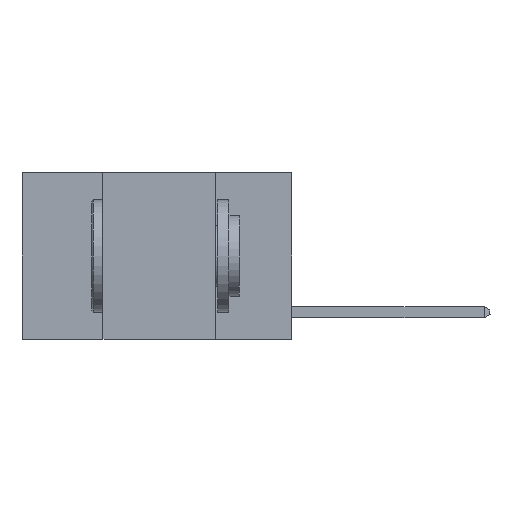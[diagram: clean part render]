
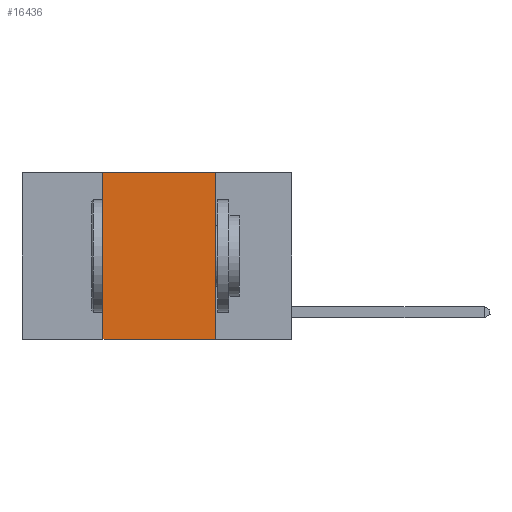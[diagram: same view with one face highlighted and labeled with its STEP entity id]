
A CAD part, left-side view. The second image highlights one B-rep face of the part: STEP entity #16436.
In plain terms, the highlighted planar face has unit normal (-1, 0, 0).
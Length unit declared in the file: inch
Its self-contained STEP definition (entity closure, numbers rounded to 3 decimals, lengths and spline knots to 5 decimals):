
#445 = VECTOR ( 'NONE', #25201, 39.37008 ) ;
#454 = ORIENTED_EDGE ( 'NONE', *, *, #23376, .F. ) ;
#1463 = PLANE ( 'NONE',  #14827 ) ;
#1881 = EDGE_CURVE ( 'NONE', #23136, #19070, #21508, .T. ) ;
#3064 = VERTEX_POINT ( 'NONE', #17737 ) ;
#4097 = LINE ( 'NONE', #4528, #22938 ) ;
#4528 = CARTESIAN_POINT ( 'NONE',  ( 0., 0.6, -0.37 ) ) ;
#6183 = VECTOR ( 'NONE', #24959, 39.37008 ) ;
#6188 = CARTESIAN_POINT ( 'NONE',  ( 0., 0.6, 0. ) ) ;
#7070 = ORIENTED_EDGE ( 'NONE', *, *, #15019, .T. ) ;
#8192 = CARTESIAN_POINT ( 'NONE',  ( 0., 0.17, -0.37 ) ) ;
#10512 = EDGE_CURVE ( 'NONE', #3064, #15084, #11759, .T. ) ;
#10969 = ORIENTED_EDGE ( 'NONE', *, *, #10512, .F. ) ;
#11759 = LINE ( 'NONE', #22546, #445 ) ;
#12192 = CARTESIAN_POINT ( 'NONE',  ( 0., 0.42, 0. ) ) ;
#13046 = DIRECTION ( 'NONE',  ( 1., 0., 0. ) ) ;
#14827 = AXIS2_PLACEMENT_3D ( 'NONE', #6188, #13046, #22053 ) ;
#15019 = EDGE_CURVE ( 'NONE', #3064, #19070, #4097, .T. ) ;
#15084 = VERTEX_POINT ( 'NONE', #12192 ) ;
#15989 = DIRECTION ( 'NONE',  ( 0., -1., 0. ) ) ;
#16436 = ADVANCED_FACE ( 'NONE', ( #26482 ), #1463, .F. ) ;
#17418 = ORIENTED_EDGE ( 'NONE', *, *, #1881, .F. ) ;
#17737 = CARTESIAN_POINT ( 'NONE',  ( 0., 0.42, -0.37 ) ) ;
#18184 = CARTESIAN_POINT ( 'NONE',  ( 0., 0.6, 0. ) ) ;
#19070 = VERTEX_POINT ( 'NONE', #8192 ) ;
#19665 = CARTESIAN_POINT ( 'NONE',  ( 0., 0.17, 0. ) ) ;
#20391 = LINE ( 'NONE', #18184, #6183 ) ;
#21508 = LINE ( 'NONE', #25485, #25277 ) ;
#22053 = DIRECTION ( 'NONE',  ( 0., 0., -1. ) ) ;
#22546 = CARTESIAN_POINT ( 'NONE',  ( 0., 0.42, 0. ) ) ;
#22894 = EDGE_LOOP ( 'NONE', ( #17418, #454, #10969, #7070 ) ) ;
#22938 = VECTOR ( 'NONE', #15989, 39.37008 ) ;
#23136 = VERTEX_POINT ( 'NONE', #19665 ) ;
#23376 = EDGE_CURVE ( 'NONE', #15084, #23136, #20391, .T. ) ;
#24959 = DIRECTION ( 'NONE',  ( 0., -1., 0. ) ) ;
#25201 = DIRECTION ( 'NONE',  ( 0., 0., 1. ) ) ;
#25277 = VECTOR ( 'NONE', #27839, 39.37008 ) ;
#25485 = CARTESIAN_POINT ( 'NONE',  ( 0., 0.17, 0. ) ) ;
#26482 = FACE_OUTER_BOUND ( 'NONE', #22894, .T. ) ;
#27839 = DIRECTION ( 'NONE',  ( 0., 0., -1. ) ) ;
